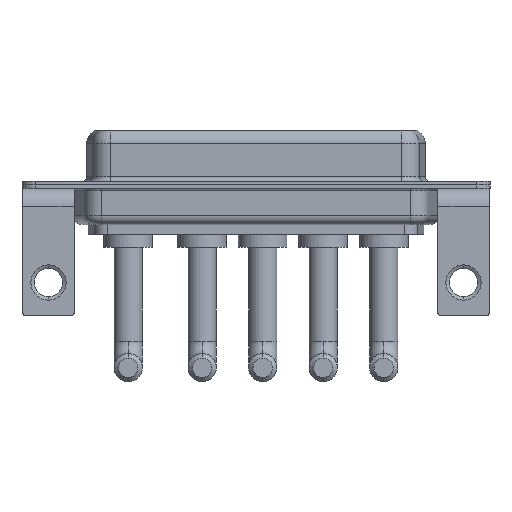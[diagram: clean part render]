
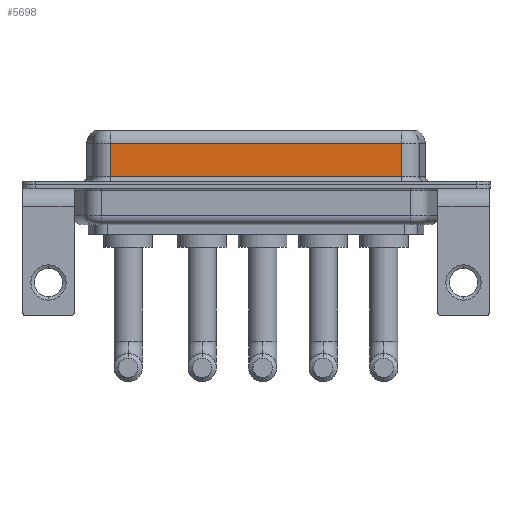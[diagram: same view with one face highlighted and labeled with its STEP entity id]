
A CAD part, front view. The second image highlights one B-rep face of the part: STEP entity #5698.
In plain terms, the highlighted planar face has unit normal (0, -1, 0).
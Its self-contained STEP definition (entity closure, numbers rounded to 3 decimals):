
#91 = EDGE_CURVE ( 'NONE', #7803, #7727, #5890, .T. ) ;
#748 = EDGE_CURVE ( 'NONE', #3515, #7727, #6528, .T. ) ;
#1387 = VECTOR ( 'NONE', #11066, 1000. ) ;
#1794 = LINE ( 'NONE', #8059, #8822 ) ;
#1871 = DIRECTION ( 'NONE',  ( -1., 0., 0. ) ) ;
#2804 = CARTESIAN_POINT ( 'NONE',  ( 7.013, -3.95, 0.9 ) ) ;
#3404 = CARTESIAN_POINT ( 'NONE',  ( 40.037, -3.95, 6.4 ) ) ;
#3515 = VERTEX_POINT ( 'NONE', #6910 ) ;
#3909 = DIRECTION ( 'NONE',  ( 0., 0., -1. ) ) ;
#4114 = DIRECTION ( 'NONE',  ( 0., 1., 0. ) ) ;
#4144 = CARTESIAN_POINT ( 'NONE',  ( 7.013, -3.95, 4.65 ) ) ;
#4350 = VERTEX_POINT ( 'NONE', #4144 ) ;
#4536 = ORIENTED_EDGE ( 'NONE', *, *, #748, .F. ) ;
#5231 = AXIS2_PLACEMENT_3D ( 'NONE', #6418, #4114, #9420 ) ;
#5413 = FACE_OUTER_BOUND ( 'NONE', #9939, .T. ) ;
#5475 = EDGE_CURVE ( 'NONE', #3515, #4350, #6093, .T. ) ;
#5698 = ADVANCED_FACE ( 'NONE', ( #5413 ), #9558, .F. ) ;
#5818 = VECTOR ( 'NONE', #10689, 1000. ) ;
#5890 = LINE ( 'NONE', #10088, #1387 ) ;
#6093 = LINE ( 'NONE', #7109, #6094 ) ;
#6094 = VECTOR ( 'NONE', #1871, 1000. ) ;
#6418 = CARTESIAN_POINT ( 'NONE',  ( 40.037, -3.95, 6.4 ) ) ;
#6528 = LINE ( 'NONE', #3404, #5818 ) ;
#6829 = ORIENTED_EDGE ( 'NONE', *, *, #5475, .T. ) ;
#6910 = CARTESIAN_POINT ( 'NONE',  ( 40.037, -3.95, 4.65 ) ) ;
#7109 = CARTESIAN_POINT ( 'NONE',  ( 40.037, -3.95, 4.65 ) ) ;
#7727 = VERTEX_POINT ( 'NONE', #12990 ) ;
#7803 = VERTEX_POINT ( 'NONE', #2804 ) ;
#8059 = CARTESIAN_POINT ( 'NONE',  ( 7.013, -3.95, 6.4 ) ) ;
#8822 = VECTOR ( 'NONE', #3909, 1000. ) ;
#9420 = DIRECTION ( 'NONE',  ( 0., 0., 1. ) ) ;
#9558 = PLANE ( 'NONE',  #5231 ) ;
#9939 = EDGE_LOOP ( 'NONE', ( #4536, #6829, #12934, #12323 ) ) ;
#10088 = CARTESIAN_POINT ( 'NONE',  ( 40.037, -3.95, 0.9 ) ) ;
#10689 = DIRECTION ( 'NONE',  ( 0., 0., -1. ) ) ;
#11066 = DIRECTION ( 'NONE',  ( 1., 0., 0. ) ) ;
#12323 = ORIENTED_EDGE ( 'NONE', *, *, #91, .T. ) ;
#12797 = EDGE_CURVE ( 'NONE', #4350, #7803, #1794, .T. ) ;
#12934 = ORIENTED_EDGE ( 'NONE', *, *, #12797, .T. ) ;
#12990 = CARTESIAN_POINT ( 'NONE',  ( 40.037, -3.95, 0.9 ) ) ;
